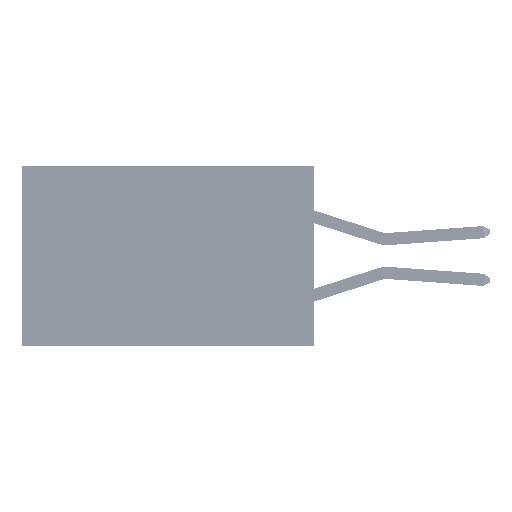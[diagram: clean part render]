
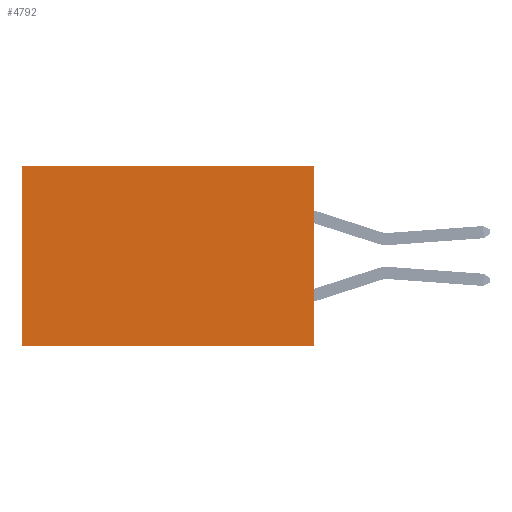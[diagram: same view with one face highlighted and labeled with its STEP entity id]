
A CAD part, left-side view. The second image highlights one B-rep face of the part: STEP entity #4792.
In plain terms, the highlighted planar face has unit normal (-1, 0, 0).
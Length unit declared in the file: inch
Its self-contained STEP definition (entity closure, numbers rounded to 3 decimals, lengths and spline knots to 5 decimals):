
#673 = PLANE ( 'NONE',  #20068 ) ;
#811 = VERTEX_POINT ( 'NONE', #36179 ) ;
#852 = EDGE_CURVE ( 'NONE', #1347, #811, #5067, .T. ) ;
#1276 = DIRECTION ( 'NONE',  ( 0., 0., -1. ) ) ;
#1347 = VERTEX_POINT ( 'NONE', #32861 ) ;
#1930 = CARTESIAN_POINT ( 'NONE',  ( 0.2875, 0., 0. ) ) ;
#4227 = CARTESIAN_POINT ( 'NONE',  ( 0.2875, 0., -0.37 ) ) ;
#4789 = DIRECTION ( 'NONE',  ( 1., 0., 0. ) ) ;
#4792 = ADVANCED_FACE ( 'NONE', ( #7771 ), #673, .F. ) ;
#5067 = LINE ( 'NONE', #11691, #36865 ) ;
#7007 = VECTOR ( 'NONE', #24140, 39.37008 ) ;
#7771 = FACE_OUTER_BOUND ( 'NONE', #41427, .T. ) ;
#11691 = CARTESIAN_POINT ( 'NONE',  ( 0.2875, 0.6, 0. ) ) ;
#13225 = LINE ( 'NONE', #1930, #31853 ) ;
#14460 = ORIENTED_EDGE ( 'NONE', *, *, #21216, .T. ) ;
#16707 = CARTESIAN_POINT ( 'NONE',  ( 0.2875, 0., 0. ) ) ;
#16889 = VERTEX_POINT ( 'NONE', #21633 ) ;
#17908 = EDGE_CURVE ( 'NONE', #28619, #811, #49291, .T. ) ;
#19019 = ORIENTED_EDGE ( 'NONE', *, *, #852, .T. ) ;
#19787 = ORIENTED_EDGE ( 'NONE', *, *, #17908, .F. ) ;
#20068 = AXIS2_PLACEMENT_3D ( 'NONE', #16707, #4789, #32678 ) ;
#20348 = CARTESIAN_POINT ( 'NONE',  ( 0.2875, 0., -0.37 ) ) ;
#20633 = CARTESIAN_POINT ( 'NONE',  ( 0.2875, 0., 0. ) ) ;
#21216 = EDGE_CURVE ( 'NONE', #16889, #1347, #51450, .T. ) ;
#21633 = CARTESIAN_POINT ( 'NONE',  ( 0.2875, 0., 0. ) ) ;
#24140 = DIRECTION ( 'NONE',  ( 0., 1., 0. ) ) ;
#28619 = VERTEX_POINT ( 'NONE', #20348 ) ;
#31853 = VECTOR ( 'NONE', #45834, 39.37008 ) ;
#32627 = DIRECTION ( 'NONE',  ( 0., 1., 0. ) ) ;
#32678 = DIRECTION ( 'NONE',  ( 0., 0., -1. ) ) ;
#32861 = CARTESIAN_POINT ( 'NONE',  ( 0.2875, 0.6, 0. ) ) ;
#34928 = EDGE_CURVE ( 'NONE', #16889, #28619, #13225, .T. ) ;
#36179 = CARTESIAN_POINT ( 'NONE',  ( 0.2875, 0.6, -0.37 ) ) ;
#36865 = VECTOR ( 'NONE', #1276, 39.37008 ) ;
#40972 = VECTOR ( 'NONE', #32627, 39.37008 ) ;
#41427 = EDGE_LOOP ( 'NONE', ( #19019, #19787, #47447, #14460 ) ) ;
#45834 = DIRECTION ( 'NONE',  ( 0., 0., -1. ) ) ;
#47447 = ORIENTED_EDGE ( 'NONE', *, *, #34928, .F. ) ;
#49291 = LINE ( 'NONE', #4227, #7007 ) ;
#51450 = LINE ( 'NONE', #20633, #40972 ) ;
